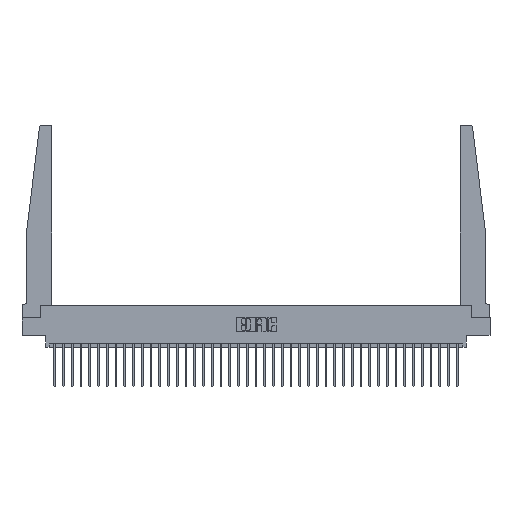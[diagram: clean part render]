
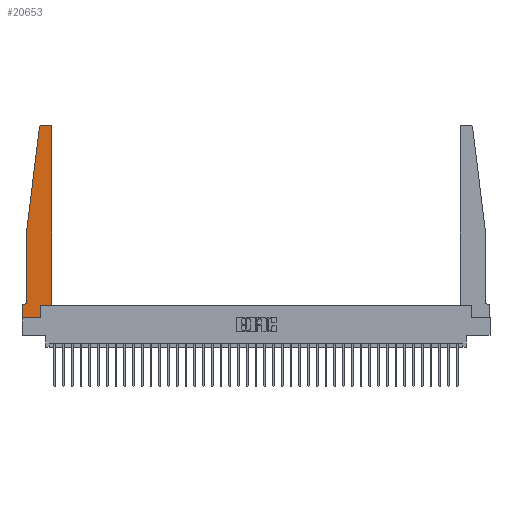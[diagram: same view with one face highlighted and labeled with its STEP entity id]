
A CAD part, top view. The second image highlights one B-rep face of the part: STEP entity #20653.
In plain terms, the highlighted planar face has unit normal (0, 0, 1).
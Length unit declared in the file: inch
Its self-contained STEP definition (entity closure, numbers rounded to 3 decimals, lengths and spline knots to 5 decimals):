
#376 = DIRECTION ( 'NONE',  ( 0., 0., -1. ) ) ;
#599 = VERTEX_POINT ( 'NONE', #30728 ) ;
#890 = DIRECTION ( 'NONE',  ( 0., -1., 0. ) ) ;
#1396 = CARTESIAN_POINT ( 'NONE',  ( 0., 0.1875, 0.37 ) ) ;
#1891 = EDGE_CURVE ( 'NONE', #13211, #31068, #18285, .T. ) ;
#1984 = CARTESIAN_POINT ( 'NONE',  ( 0.25, 2.75, 0.37 ) ) ;
#2400 = LINE ( 'NONE', #8318, #20674 ) ;
#2455 = AXIS2_PLACEMENT_3D ( 'NONE', #13622, #10939, #11463 ) ;
#2504 = VECTOR ( 'NONE', #17915, 39.37008 ) ;
#2908 = DIRECTION ( 'NONE',  ( -1., 0., 0. ) ) ;
#2979 = DIRECTION ( 'NONE',  ( 0., 1., 0. ) ) ;
#3005 = CARTESIAN_POINT ( 'NONE',  ( 0.24675, 2.72367, 0.37 ) ) ;
#4073 = VECTOR ( 'NONE', #28075, 39.37008 ) ;
#4395 = EDGE_CURVE ( 'NONE', #27364, #13211, #15582, .T. ) ;
#4516 = ORIENTED_EDGE ( 'NONE', *, *, #7424, .T. ) ;
#4966 = ORIENTED_EDGE ( 'NONE', *, *, #28375, .T. ) ;
#5081 = DIRECTION ( 'NONE',  ( 0., -1., 0. ) ) ;
#5322 = VERTEX_POINT ( 'NONE', #16524 ) ;
#5481 = DIRECTION ( 'NONE',  ( 0., 0., 1. ) ) ;
#5606 = ORIENTED_EDGE ( 'NONE', *, *, #13365, .T. ) ;
#6876 = EDGE_CURVE ( 'NONE', #9115, #27364, #14450, .T. ) ;
#7424 = EDGE_CURVE ( 'NONE', #21150, #599, #30600, .T. ) ;
#8260 = VERTEX_POINT ( 'NONE', #33686 ) ;
#8318 = CARTESIAN_POINT ( 'NONE',  ( 0., 0., 0.37 ) ) ;
#8730 = CARTESIAN_POINT ( 'NONE',  ( 0.2605, 0.18, 0.37 ) ) ;
#8949 = ORIENTED_EDGE ( 'NONE', *, *, #34453, .T. ) ;
#9115 = VERTEX_POINT ( 'NONE', #12734 ) ;
#9581 = EDGE_CURVE ( 'NONE', #5322, #30714, #34049, .T. ) ;
#9937 = CARTESIAN_POINT ( 'NONE',  ( 0.425, 0.18, 0.37 ) ) ;
#10113 = DIRECTION ( 'NONE',  ( 1., 0., 0. ) ) ;
#10939 = DIRECTION ( 'NONE',  ( 0., 0., 1. ) ) ;
#11463 = DIRECTION ( 'NONE',  ( 1., 0., 0. ) ) ;
#11995 = AXIS2_PLACEMENT_3D ( 'NONE', #30912, #33780, #26068 ) ;
#12153 = EDGE_LOOP ( 'NONE', ( #33891, #30052, #34890, #4516, #4966, #30403, #5606, #34908, #14027, #16899, #8949, #13118 ) ) ;
#12278 = CARTESIAN_POINT ( 'NONE',  ( 0.27653, 2.75, 0.37 ) ) ;
#12726 = EDGE_CURVE ( 'NONE', #30714, #31863, #28265, .T. ) ;
#12734 = CARTESIAN_POINT ( 'NONE',  ( 0.425, 2.72, 0.37 ) ) ;
#13060 = CARTESIAN_POINT ( 'NONE',  ( 0.015, 0.1875, 0.37 ) ) ;
#13118 = ORIENTED_EDGE ( 'NONE', *, *, #6876, .T. ) ;
#13211 = VERTEX_POINT ( 'NONE', #12278 ) ;
#13365 = EDGE_CURVE ( 'NONE', #28955, #5322, #2400, .T. ) ;
#13622 = CARTESIAN_POINT ( 'NONE',  ( 0.395, 2.72, 0.37 ) ) ;
#14004 = VECTOR ( 'NONE', #2979, 39.37008 ) ;
#14027 = ORIENTED_EDGE ( 'NONE', *, *, #12726, .T. ) ;
#14450 = CIRCLE ( 'NONE', #2455, 0.03 ) ;
#14568 = VECTOR ( 'NONE', #10113, 39.37008 ) ;
#15582 = LINE ( 'NONE', #1984, #26328 ) ;
#15655 = CARTESIAN_POINT ( 'NONE',  ( 0.2605, 0.18, 0.37 ) ) ;
#15916 = AXIS2_PLACEMENT_3D ( 'NONE', #34865, #5481, #24452 ) ;
#16211 = FACE_OUTER_BOUND ( 'NONE', #12153, .T. ) ;
#16524 = CARTESIAN_POINT ( 'NONE',  ( 0., 0., 0.37 ) ) ;
#16899 = ORIENTED_EDGE ( 'NONE', *, *, #31736, .T. ) ;
#17022 = VECTOR ( 'NONE', #32434, 39.37008 ) ;
#17159 = CARTESIAN_POINT ( 'NONE',  ( 0.065, 1.25, 0.37 ) ) ;
#17366 = DIRECTION ( 'NONE',  ( -1., 0., 0. ) ) ;
#17432 = VERTEX_POINT ( 'NONE', #13060 ) ;
#17915 = DIRECTION ( 'NONE',  ( 1., 0., 0. ) ) ;
#18285 = CIRCLE ( 'NONE', #11995, 0.03 ) ;
#19172 = CARTESIAN_POINT ( 'NONE',  ( 0.065, 1.25, 0.37 ) ) ;
#19303 = EDGE_CURVE ( 'NONE', #17432, #28955, #24935, .T. ) ;
#19633 = LINE ( 'NONE', #21965, #14004 ) ;
#19767 = EDGE_CURVE ( 'NONE', #31068, #21150, #32258, .T. ) ;
#20653 = ADVANCED_FACE ( 'NONE', ( #16211 ), #29474, .T. ) ;
#20674 = VECTOR ( 'NONE', #5081, 39.37008 ) ;
#21150 = VERTEX_POINT ( 'NONE', #31498 ) ;
#21965 = CARTESIAN_POINT ( 'NONE',  ( 0.425, 0.18, 0.37 ) ) ;
#24452 = DIRECTION ( 'NONE',  ( 1., 0., 0. ) ) ;
#24935 = LINE ( 'NONE', #30129, #27155 ) ;
#25062 = CARTESIAN_POINT ( 'NONE',  ( 0.015, 0.2375, 0.37 ) ) ;
#25781 = CARTESIAN_POINT ( 'NONE',  ( 0., 0., 0.37 ) ) ;
#26068 = DIRECTION ( 'NONE',  ( 1., 0., 0. ) ) ;
#26328 = VECTOR ( 'NONE', #29720, 39.37008 ) ;
#26395 = LINE ( 'NONE', #9937, #14568 ) ;
#27155 = VECTOR ( 'NONE', #2908, 39.37008 ) ;
#27280 = CARTESIAN_POINT ( 'NONE',  ( 0.2605, 0., 0.37 ) ) ;
#27364 = VERTEX_POINT ( 'NONE', #32202 ) ;
#27638 = AXIS2_PLACEMENT_3D ( 'NONE', #25062, #376, #17366 ) ;
#28075 = DIRECTION ( 'NONE',  ( 0., 1., 0. ) ) ;
#28265 = LINE ( 'NONE', #8730, #4073 ) ;
#28375 = EDGE_CURVE ( 'NONE', #599, #17432, #32233, .T. ) ;
#28955 = VERTEX_POINT ( 'NONE', #1396 ) ;
#29474 = PLANE ( 'NONE',  #15916 ) ;
#29720 = DIRECTION ( 'NONE',  ( -1., 0., 0. ) ) ;
#30052 = ORIENTED_EDGE ( 'NONE', *, *, #1891, .T. ) ;
#30129 = CARTESIAN_POINT ( 'NONE',  ( 0.065, 0.1875, 0.37 ) ) ;
#30403 = ORIENTED_EDGE ( 'NONE', *, *, #19303, .T. ) ;
#30600 = LINE ( 'NONE', #17159, #34534 ) ;
#30714 = VERTEX_POINT ( 'NONE', #27280 ) ;
#30728 = CARTESIAN_POINT ( 'NONE',  ( 0.065, 0.2375, 0.37 ) ) ;
#30912 = CARTESIAN_POINT ( 'NONE',  ( 0.27653, 2.72, 0.37 ) ) ;
#31068 = VERTEX_POINT ( 'NONE', #3005 ) ;
#31498 = CARTESIAN_POINT ( 'NONE',  ( 0.065, 1.25, 0.37 ) ) ;
#31736 = EDGE_CURVE ( 'NONE', #31863, #8260, #26395, .T. ) ;
#31863 = VERTEX_POINT ( 'NONE', #15655 ) ;
#32202 = CARTESIAN_POINT ( 'NONE',  ( 0.395, 2.75, 0.37 ) ) ;
#32233 = CIRCLE ( 'NONE', #27638, 0.05 ) ;
#32258 = LINE ( 'NONE', #19172, #17022 ) ;
#32434 = DIRECTION ( 'NONE',  ( -0.122, -0.992, 0. ) ) ;
#33686 = CARTESIAN_POINT ( 'NONE',  ( 0.425, 0.18, 0.37 ) ) ;
#33780 = DIRECTION ( 'NONE',  ( 0., 0., 1. ) ) ;
#33891 = ORIENTED_EDGE ( 'NONE', *, *, #4395, .T. ) ;
#34049 = LINE ( 'NONE', #25781, #2504 ) ;
#34453 = EDGE_CURVE ( 'NONE', #8260, #9115, #19633, .T. ) ;
#34534 = VECTOR ( 'NONE', #890, 39.37008 ) ;
#34865 = CARTESIAN_POINT ( 'NONE',  ( 0., 0.1875, 0.37 ) ) ;
#34890 = ORIENTED_EDGE ( 'NONE', *, *, #19767, .T. ) ;
#34908 = ORIENTED_EDGE ( 'NONE', *, *, #9581, .T. ) ;
